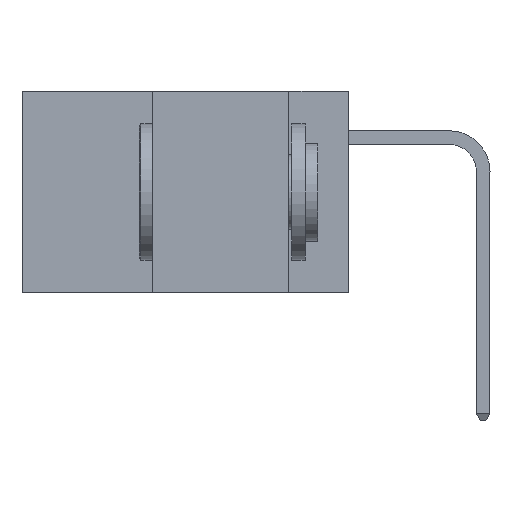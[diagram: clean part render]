
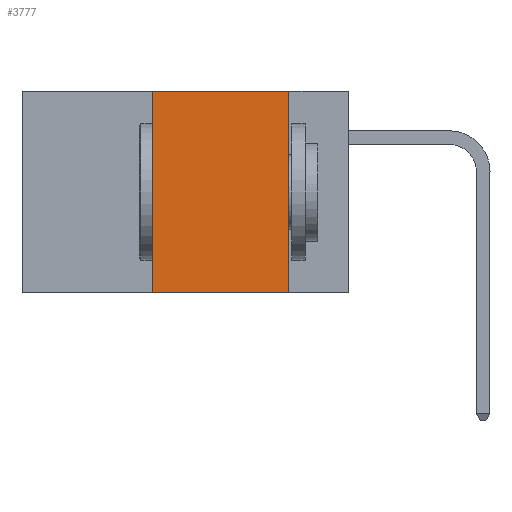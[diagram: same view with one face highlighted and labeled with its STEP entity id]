
A CAD part, left-side view. The second image highlights one B-rep face of the part: STEP entity #3777.
In plain terms, the highlighted planar face has unit normal (-1, 0, 0).
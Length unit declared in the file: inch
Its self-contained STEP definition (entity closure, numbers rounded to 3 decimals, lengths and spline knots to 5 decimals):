
#197 = EDGE_CURVE ( 'NONE', #735, #28750, #1890, .T. ) ;
#735 = VERTEX_POINT ( 'NONE', #12237 ) ;
#1890 = LINE ( 'NONE', #27006, #19998 ) ;
#2214 = EDGE_CURVE ( 'NONE', #28750, #28274, #8538, .T. ) ;
#2441 = DIRECTION ( 'NONE',  ( 0., -1., 0. ) ) ;
#3295 = CARTESIAN_POINT ( 'NONE',  ( 0., 0.6, 0. ) ) ;
#3372 = ORIENTED_EDGE ( 'NONE', *, *, #2214, .F. ) ;
#3777 = ADVANCED_FACE ( 'NONE', ( #20505 ), #13712, .F. ) ;
#7495 = ORIENTED_EDGE ( 'NONE', *, *, #8272, .F. ) ;
#7989 = CARTESIAN_POINT ( 'NONE',  ( 0., 0.11, -0.37 ) ) ;
#8272 = EDGE_CURVE ( 'NONE', #28274, #11695, #23577, .T. ) ;
#8538 = LINE ( 'NONE', #3295, #19517 ) ;
#11484 = DIRECTION ( 'NONE',  ( 0., 0., -1. ) ) ;
#11695 = VERTEX_POINT ( 'NONE', #7989 ) ;
#12237 = CARTESIAN_POINT ( 'NONE',  ( 0., 0.36, -0.37 ) ) ;
#12515 = DIRECTION ( 'NONE',  ( 0., 0., 1. ) ) ;
#13351 = DIRECTION ( 'NONE',  ( 0., 0., -1. ) ) ;
#13712 = PLANE ( 'NONE',  #17599 ) ;
#14314 = CARTESIAN_POINT ( 'NONE',  ( 0., 0.6, -0.37 ) ) ;
#14595 = EDGE_CURVE ( 'NONE', #735, #11695, #26275, .T. ) ;
#17416 = ORIENTED_EDGE ( 'NONE', *, *, #197, .F. ) ;
#17599 = AXIS2_PLACEMENT_3D ( 'NONE', #23111, #25447, #11484 ) ;
#19517 = VECTOR ( 'NONE', #22160, 39.37008 ) ;
#19998 = VECTOR ( 'NONE', #12515, 39.37008 ) ;
#20027 = VECTOR ( 'NONE', #2441, 39.37008 ) ;
#20250 = CARTESIAN_POINT ( 'NONE',  ( 0., 0.11, 0. ) ) ;
#20505 = FACE_OUTER_BOUND ( 'NONE', #21269, .T. ) ;
#21269 = EDGE_LOOP ( 'NONE', ( #7495, #3372, #17416, #25127 ) ) ;
#22160 = DIRECTION ( 'NONE',  ( 0., -1., 0. ) ) ;
#22835 = VECTOR ( 'NONE', #13351, 39.37008 ) ;
#22944 = CARTESIAN_POINT ( 'NONE',  ( 0., 0.11, 0. ) ) ;
#23111 = CARTESIAN_POINT ( 'NONE',  ( 0., 0.6, 0. ) ) ;
#23577 = LINE ( 'NONE', #20250, #22835 ) ;
#25127 = ORIENTED_EDGE ( 'NONE', *, *, #14595, .T. ) ;
#25447 = DIRECTION ( 'NONE',  ( 1., 0., 0. ) ) ;
#26275 = LINE ( 'NONE', #14314, #20027 ) ;
#27006 = CARTESIAN_POINT ( 'NONE',  ( 0., 0.36, 0. ) ) ;
#28274 = VERTEX_POINT ( 'NONE', #22944 ) ;
#28750 = VERTEX_POINT ( 'NONE', #29700 ) ;
#29700 = CARTESIAN_POINT ( 'NONE',  ( 0., 0.36, 0. ) ) ;
